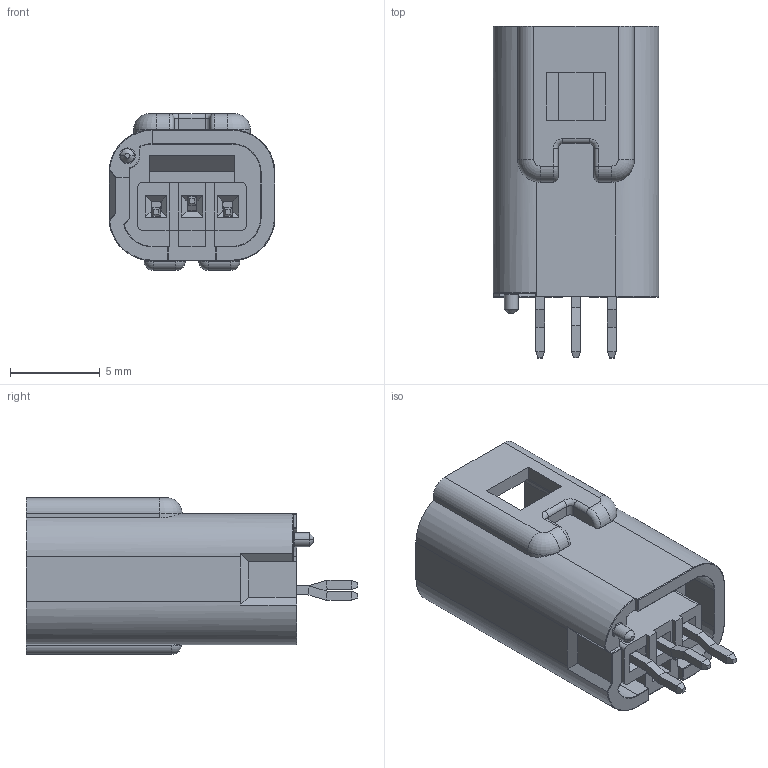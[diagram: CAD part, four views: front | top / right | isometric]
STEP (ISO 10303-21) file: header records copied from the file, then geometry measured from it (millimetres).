
FILE_DESCRIPTION (( 'STEP AP214' ), '1' );
FILE_NAME ('566-003-421-701.STEP', '2020-07-30T20:42:39', ( '' ), ( '' ), 'SwSTEP 2.0', 'SolidWorks 2020', '' );
FILE_SCHEMA (( 'AUTOMOTIVE_DESIGN' ));
Length unit declared in the file: millimetre
Products named in the file (5): 566-003-421-701_ rubber.STEP; 566-003-421-701.STEP; 566-003-421-701; 566-003-421-701_plastic.STEP; 566-003-421-701_contact.STEP
Assembly tree (6 placements, depth 3):
  566-003-421-701
    566-003-421-701.STEP
      566-003-421-701_plastic.STEP
      566-003-421-701_ rubber.STEP
      566-003-421-701_contact.STEP  x3
Bounding box: 9.25 x 18.5 x 8.74 mm (x, y, z)
Volume: 508 mm3; surface area: 1397.4 mm2
Topology: 5 solids, 5 shells, 718 faces, 1676 edges, 982 vertices
Faces by surface type: plane 304, cylinder 231, torus 155, cone 16, sphere 12
Entity records: 18835 total; most frequent: CARTESIAN_POINT 3824, DIRECTION 3283, ORIENTED_EDGE 3016, EDGE_CURVE 1508, AXIS2_PLACEMENT_3D 1198, VERTEX_POINT 890, LINE 887, VECTOR 887
